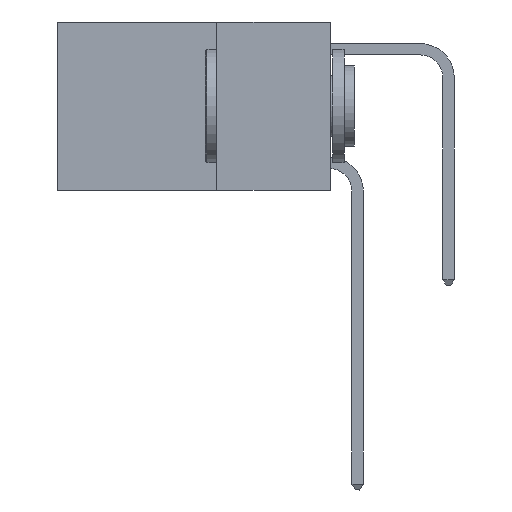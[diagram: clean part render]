
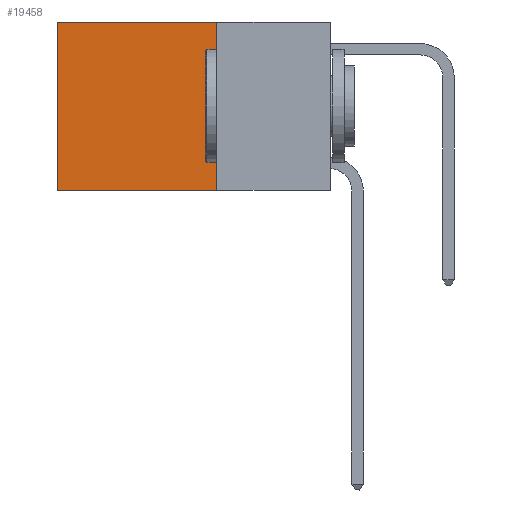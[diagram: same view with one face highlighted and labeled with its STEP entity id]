
A CAD part, left-side view. The second image highlights one B-rep face of the part: STEP entity #19458.
In plain terms, the highlighted planar face has unit normal (-1, 0, 0).
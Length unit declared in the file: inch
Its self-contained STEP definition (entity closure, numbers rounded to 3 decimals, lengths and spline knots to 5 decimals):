
#460 = LINE ( 'NONE', #23148, #22526 ) ;
#1098 = CARTESIAN_POINT ( 'NONE',  ( 0.2625, 0.6, 0. ) ) ;
#1223 = CARTESIAN_POINT ( 'NONE',  ( 0.2625, 0.6, -0.37 ) ) ;
#1540 = VERTEX_POINT ( 'NONE', #1223 ) ;
#1695 = VERTEX_POINT ( 'NONE', #14637 ) ;
#2184 = ORIENTED_EDGE ( 'NONE', *, *, #19240, .T. ) ;
#4483 = CARTESIAN_POINT ( 'NONE',  ( 0.2625, 0.25, 0. ) ) ;
#4580 = EDGE_CURVE ( 'NONE', #9332, #11606, #460, .T. ) ;
#4694 = DIRECTION ( 'NONE',  ( 0., 1., 0. ) ) ;
#4724 = EDGE_CURVE ( 'NONE', #1695, #1540, #18258, .T. ) ;
#5288 = DIRECTION ( 'NONE',  ( 1., 0., 0. ) ) ;
#8457 = LINE ( 'NONE', #4483, #20969 ) ;
#9332 = VERTEX_POINT ( 'NONE', #23958 ) ;
#10865 = LINE ( 'NONE', #21311, #21595 ) ;
#10921 = DIRECTION ( 'NONE',  ( 0., 0., -1. ) ) ;
#11183 = PLANE ( 'NONE',  #20556 ) ;
#11606 = VERTEX_POINT ( 'NONE', #11627 ) ;
#11627 = CARTESIAN_POINT ( 'NONE',  ( 0.2625, 0.25, -0.37 ) ) ;
#12823 = ORIENTED_EDGE ( 'NONE', *, *, #25703, .F. ) ;
#14637 = CARTESIAN_POINT ( 'NONE',  ( 0.2625, 0.6, 0. ) ) ;
#16472 = ORIENTED_EDGE ( 'NONE', *, *, #4580, .F. ) ;
#16717 = DIRECTION ( 'NONE',  ( 0., 1., 0. ) ) ;
#17785 = CARTESIAN_POINT ( 'NONE',  ( 0.2625, 0.25, 0. ) ) ;
#18258 = LINE ( 'NONE', #1098, #21205 ) ;
#19240 = EDGE_CURVE ( 'NONE', #9332, #1695, #8457, .T. ) ;
#19436 = EDGE_LOOP ( 'NONE', ( #20608, #12823, #16472, #2184 ) ) ;
#19458 = ADVANCED_FACE ( 'NONE', ( #23867 ), #11183, .F. ) ;
#20556 = AXIS2_PLACEMENT_3D ( 'NONE', #17785, #5288, #25482 ) ;
#20608 = ORIENTED_EDGE ( 'NONE', *, *, #4724, .T. ) ;
#20969 = VECTOR ( 'NONE', #16717, 39.37008 ) ;
#21205 = VECTOR ( 'NONE', #26377, 39.37008 ) ;
#21311 = CARTESIAN_POINT ( 'NONE',  ( 0.2625, 0.25, -0.37 ) ) ;
#21595 = VECTOR ( 'NONE', #4694, 39.37008 ) ;
#22526 = VECTOR ( 'NONE', #10921, 39.37008 ) ;
#23148 = CARTESIAN_POINT ( 'NONE',  ( 0.2625, 0.25, 0. ) ) ;
#23867 = FACE_OUTER_BOUND ( 'NONE', #19436, .T. ) ;
#23958 = CARTESIAN_POINT ( 'NONE',  ( 0.2625, 0.25, 0. ) ) ;
#25482 = DIRECTION ( 'NONE',  ( 0., 0., -1. ) ) ;
#25703 = EDGE_CURVE ( 'NONE', #11606, #1540, #10865, .T. ) ;
#26377 = DIRECTION ( 'NONE',  ( 0., 0., -1. ) ) ;
